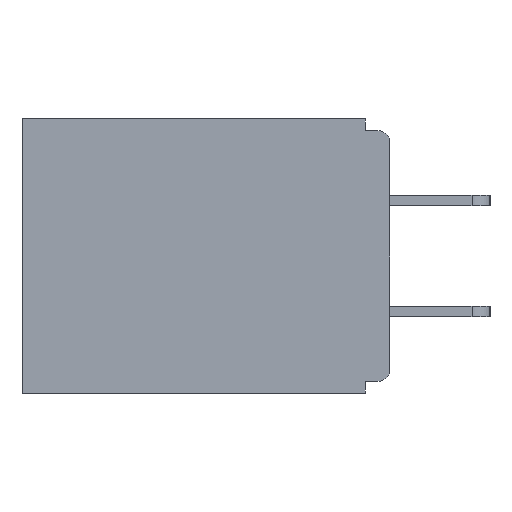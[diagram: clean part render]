
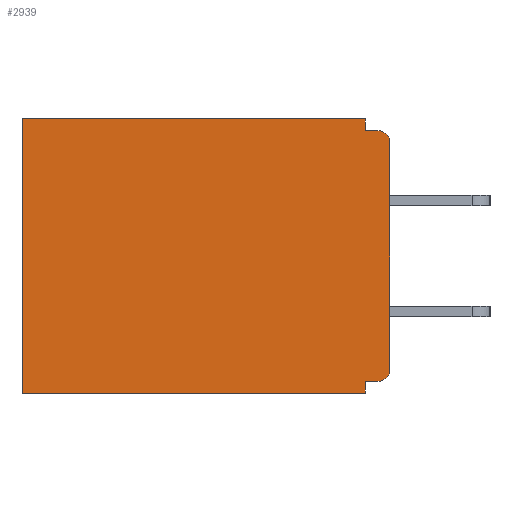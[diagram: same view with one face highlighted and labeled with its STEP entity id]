
A CAD part, left-side view. The second image highlights one B-rep face of the part: STEP entity #2939.
In plain terms, the highlighted planar face has unit normal (-1, 0, 0).
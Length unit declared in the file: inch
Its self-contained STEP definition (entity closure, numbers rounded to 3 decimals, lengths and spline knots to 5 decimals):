
#27 = ORIENTED_EDGE ( 'NONE', *, *, #18175, .F. ) ;
#66 = VERTEX_POINT ( 'NONE', #4985 ) ;
#99 = AXIS2_PLACEMENT_3D ( 'NONE', #13061, #4533, #3204 ) ;
#201 = VERTEX_POINT ( 'NONE', #15224 ) ;
#221 = VECTOR ( 'NONE', #11715, 39.37008 ) ;
#697 = ORIENTED_EDGE ( 'NONE', *, *, #14528, .F. ) ;
#1014 = VERTEX_POINT ( 'NONE', #6395 ) ;
#1417 = DIRECTION ( 'NONE',  ( 0., 0., -1. ) ) ;
#1606 = CARTESIAN_POINT ( 'NONE',  ( 0.298, 0., -0.328 ) ) ;
#1621 = VECTOR ( 'NONE', #2289, 39.37008 ) ;
#1908 = CARTESIAN_POINT ( 'NONE',  ( 0.298, 0.015, -0.313 ) ) ;
#2289 = DIRECTION ( 'NONE',  ( 0., 0., -1. ) ) ;
#2307 = VECTOR ( 'NONE', #8986, 39.37008 ) ;
#2461 = LINE ( 'NONE', #4128, #6605 ) ;
#2555 = LINE ( 'NONE', #3745, #15253 ) ;
#2939 = ADVANCED_FACE ( 'NONE', ( #5222 ), #7597, .F. ) ;
#3142 = CARTESIAN_POINT ( 'NONE',  ( 0.298, 0., -0.343 ) ) ;
#3204 = DIRECTION ( 'NONE',  ( 0., 0., -1. ) ) ;
#3745 = CARTESIAN_POINT ( 'NONE',  ( 0.298, 0., -0.015 ) ) ;
#3799 = DIRECTION ( 'NONE',  ( 0., -1., 0. ) ) ;
#4128 = CARTESIAN_POINT ( 'NONE',  ( 0.298, 0., 0. ) ) ;
#4132 = EDGE_CURVE ( 'NONE', #5521, #17431, #2555, .T. ) ;
#4430 = LINE ( 'NONE', #12002, #1621 ) ;
#4533 = DIRECTION ( 'NONE',  ( -1., 0., 0. ) ) ;
#4686 = VERTEX_POINT ( 'NONE', #16451 ) ;
#4697 = LINE ( 'NONE', #3142, #15900 ) ;
#4743 = AXIS2_PLACEMENT_3D ( 'NONE', #1908, #6171, #13147 ) ;
#4985 = CARTESIAN_POINT ( 'NONE',  ( 0.298, 0., -0.03 ) ) ;
#5009 = ORIENTED_EDGE ( 'NONE', *, *, #16426, .T. ) ;
#5013 = EDGE_CURVE ( 'NONE', #201, #5450, #13900, .T. ) ;
#5200 = ORIENTED_EDGE ( 'NONE', *, *, #7868, .T. ) ;
#5222 = FACE_OUTER_BOUND ( 'NONE', #13669, .T. ) ;
#5450 = VERTEX_POINT ( 'NONE', #15825 ) ;
#5521 = VERTEX_POINT ( 'NONE', #10498 ) ;
#5718 = DIRECTION ( 'NONE',  ( 0., 1., 0. ) ) ;
#6171 = DIRECTION ( 'NONE',  ( -1., 0., 0. ) ) ;
#6193 = CARTESIAN_POINT ( 'NONE',  ( 0.298, 0., 0. ) ) ;
#6232 = CARTESIAN_POINT ( 'NONE',  ( 0.298, 0.031, -0.343 ) ) ;
#6395 = CARTESIAN_POINT ( 'NONE',  ( 0.298, 0.015, -0.328 ) ) ;
#6605 = VECTOR ( 'NONE', #1417, 39.37008 ) ;
#7597 = PLANE ( 'NONE',  #17795 ) ;
#7720 = DIRECTION ( 'NONE',  ( 0., 0., -1. ) ) ;
#7749 = CARTESIAN_POINT ( 'NONE',  ( 0.298, 0.031, -0.328 ) ) ;
#7868 = EDGE_CURVE ( 'NONE', #66, #17431, #16759, .T. ) ;
#8986 = DIRECTION ( 'NONE',  ( 0., 0., -1. ) ) ;
#9022 = CARTESIAN_POINT ( 'NONE',  ( 0.298, 0., 0. ) ) ;
#9382 = EDGE_CURVE ( 'NONE', #15170, #16485, #4430, .T. ) ;
#9573 = ORIENTED_EDGE ( 'NONE', *, *, #10716, .F. ) ;
#9831 = CIRCLE ( 'NONE', #4743, 0.015 ) ;
#9843 = CARTESIAN_POINT ( 'NONE',  ( 0.298, 0.031, -0.343 ) ) ;
#9881 = LINE ( 'NONE', #1606, #10088 ) ;
#10088 = VECTOR ( 'NONE', #14206, 39.37008 ) ;
#10156 = ORIENTED_EDGE ( 'NONE', *, *, #5013, .T. ) ;
#10498 = CARTESIAN_POINT ( 'NONE',  ( 0.298, 0.031, -0.015 ) ) ;
#10716 = EDGE_CURVE ( 'NONE', #4686, #5521, #10972, .T. ) ;
#10778 = VECTOR ( 'NONE', #13298, 39.37008 ) ;
#10888 = EDGE_CURVE ( 'NONE', #66, #13823, #2461, .T. ) ;
#10972 = LINE ( 'NONE', #9843, #10778 ) ;
#11334 = ORIENTED_EDGE ( 'NONE', *, *, #15863, .T. ) ;
#11715 = DIRECTION ( 'NONE',  ( 0., 1., 0. ) ) ;
#12002 = CARTESIAN_POINT ( 'NONE',  ( 0.298, 0.031, -0.343 ) ) ;
#12217 = CARTESIAN_POINT ( 'NONE',  ( 0.298, 0.46, 0. ) ) ;
#13061 = CARTESIAN_POINT ( 'NONE',  ( 0.298, 0.015, -0.03 ) ) ;
#13121 = ORIENTED_EDGE ( 'NONE', *, *, #10888, .F. ) ;
#13147 = DIRECTION ( 'NONE',  ( 0., 0., -1. ) ) ;
#13227 = DIRECTION ( 'NONE',  ( 1., 0., 0. ) ) ;
#13298 = DIRECTION ( 'NONE',  ( 0., 0., -1. ) ) ;
#13570 = LINE ( 'NONE', #9022, #221 ) ;
#13669 = EDGE_LOOP ( 'NONE', ( #5200, #16322, #9573, #11334, #10156, #27, #14612, #697, #5009, #13121 ) ) ;
#13823 = VERTEX_POINT ( 'NONE', #15487 ) ;
#13900 = LINE ( 'NONE', #12217, #2307 ) ;
#14206 = DIRECTION ( 'NONE',  ( 0., 1., 0. ) ) ;
#14528 = EDGE_CURVE ( 'NONE', #1014, #15170, #9881, .T. ) ;
#14612 = ORIENTED_EDGE ( 'NONE', *, *, #9382, .F. ) ;
#15170 = VERTEX_POINT ( 'NONE', #7749 ) ;
#15224 = CARTESIAN_POINT ( 'NONE',  ( 0.298, 0.46, 0. ) ) ;
#15246 = CARTESIAN_POINT ( 'NONE',  ( 0.298, 0.015, -0.015 ) ) ;
#15253 = VECTOR ( 'NONE', #3799, 39.37008 ) ;
#15487 = CARTESIAN_POINT ( 'NONE',  ( 0.298, 0., -0.313 ) ) ;
#15825 = CARTESIAN_POINT ( 'NONE',  ( 0.298, 0.46, -0.343 ) ) ;
#15863 = EDGE_CURVE ( 'NONE', #4686, #201, #13570, .T. ) ;
#15900 = VECTOR ( 'NONE', #5718, 39.37008 ) ;
#16322 = ORIENTED_EDGE ( 'NONE', *, *, #4132, .F. ) ;
#16426 = EDGE_CURVE ( 'NONE', #1014, #13823, #9831, .T. ) ;
#16451 = CARTESIAN_POINT ( 'NONE',  ( 0.298, 0.031, 0. ) ) ;
#16485 = VERTEX_POINT ( 'NONE', #6232 ) ;
#16759 = CIRCLE ( 'NONE', #99, 0.015 ) ;
#17431 = VERTEX_POINT ( 'NONE', #15246 ) ;
#17795 = AXIS2_PLACEMENT_3D ( 'NONE', #6193, #13227, #7720 ) ;
#18175 = EDGE_CURVE ( 'NONE', #16485, #5450, #4697, .T. ) ;
